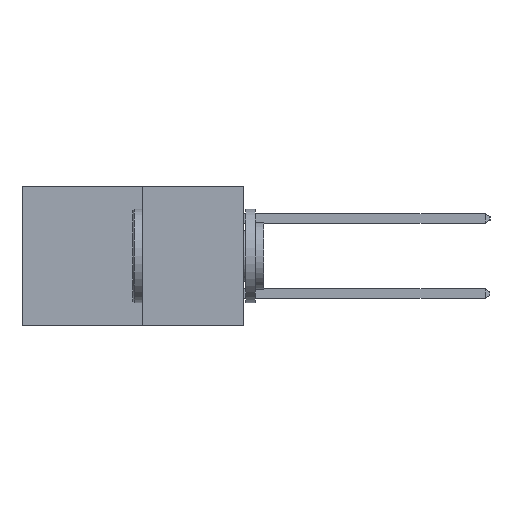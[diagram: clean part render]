
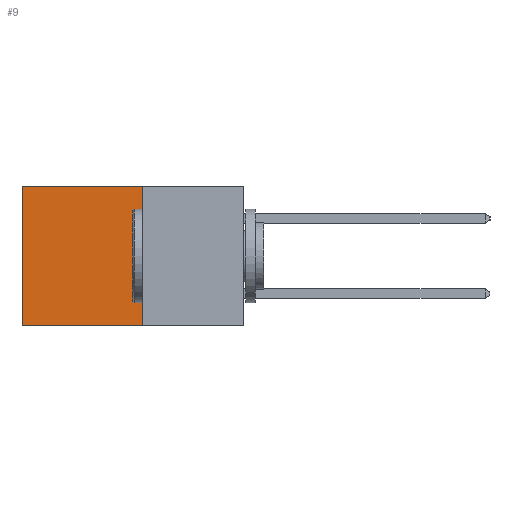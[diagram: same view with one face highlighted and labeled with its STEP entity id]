
A CAD part, left-side view. The second image highlights one B-rep face of the part: STEP entity #9.
In plain terms, the highlighted planar face has unit normal (-1, 0, 0).
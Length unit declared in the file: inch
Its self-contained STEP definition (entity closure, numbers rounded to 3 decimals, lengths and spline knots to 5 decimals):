
#9 = ADVANCED_FACE ( 'NONE', ( #10505 ), #12434, .F. ) ;
#226 = ORIENTED_EDGE ( 'NONE', *, *, #10408, .F. ) ;
#824 = DIRECTION ( 'NONE',  ( 0., 0., -1. ) ) ;
#1819 = VECTOR ( 'NONE', #824, 39.37008 ) ;
#2286 = CARTESIAN_POINT ( 'NONE',  ( 0.277, 0.27, 0. ) ) ;
#3646 = DIRECTION ( 'NONE',  ( 0., 1., 0. ) ) ;
#4049 = EDGE_CURVE ( 'NONE', #7245, #13066, #13352, .T. ) ;
#4288 = LINE ( 'NONE', #2286, #15742 ) ;
#5010 = ORIENTED_EDGE ( 'NONE', *, *, #7250, .F. ) ;
#5037 = VECTOR ( 'NONE', #3646, 39.37008 ) ;
#5076 = CARTESIAN_POINT ( 'NONE',  ( 0.277, 0.27, 0. ) ) ;
#7245 = VERTEX_POINT ( 'NONE', #12633 ) ;
#7250 = EDGE_CURVE ( 'NONE', #15815, #17174, #11279, .T. ) ;
#8093 = CARTESIAN_POINT ( 'NONE',  ( 0.277, 0.27, -0.37 ) ) ;
#8227 = CARTESIAN_POINT ( 'NONE',  ( 0.277, 0.59, -0.37 ) ) ;
#9206 = ORIENTED_EDGE ( 'NONE', *, *, #4049, .T. ) ;
#9620 = DIRECTION ( 'NONE',  ( 1., 0., 0. ) ) ;
#9898 = CARTESIAN_POINT ( 'NONE',  ( 0.277, 0.27, -0.37 ) ) ;
#10109 = DIRECTION ( 'NONE',  ( 0., 0., -1. ) ) ;
#10408 = EDGE_CURVE ( 'NONE', #17174, #13066, #12013, .T. ) ;
#10505 = FACE_OUTER_BOUND ( 'NONE', #13672, .T. ) ;
#10768 = ORIENTED_EDGE ( 'NONE', *, *, #13457, .T. ) ;
#10814 = AXIS2_PLACEMENT_3D ( 'NONE', #9898, #9620, #10109 ) ;
#11279 = LINE ( 'NONE', #12544, #14537 ) ;
#11734 = CARTESIAN_POINT ( 'NONE',  ( 0.277, 0.59, -0.37 ) ) ;
#12013 = LINE ( 'NONE', #13361, #5037 ) ;
#12290 = DIRECTION ( 'NONE',  ( 0., 0., -1. ) ) ;
#12434 = PLANE ( 'NONE',  #10814 ) ;
#12544 = CARTESIAN_POINT ( 'NONE',  ( 0.277, 0.27, -0.37 ) ) ;
#12633 = CARTESIAN_POINT ( 'NONE',  ( 0.277, 0.59, 0. ) ) ;
#13066 = VERTEX_POINT ( 'NONE', #8227 ) ;
#13352 = LINE ( 'NONE', #11734, #1819 ) ;
#13361 = CARTESIAN_POINT ( 'NONE',  ( 0.277, 0.27, -0.37 ) ) ;
#13457 = EDGE_CURVE ( 'NONE', #15815, #7245, #4288, .T. ) ;
#13672 = EDGE_LOOP ( 'NONE', ( #9206, #226, #5010, #10768 ) ) ;
#14537 = VECTOR ( 'NONE', #12290, 39.37008 ) ;
#15742 = VECTOR ( 'NONE', #17376, 39.37008 ) ;
#15815 = VERTEX_POINT ( 'NONE', #5076 ) ;
#17174 = VERTEX_POINT ( 'NONE', #8093 ) ;
#17376 = DIRECTION ( 'NONE',  ( 0., 1., 0. ) ) ;
